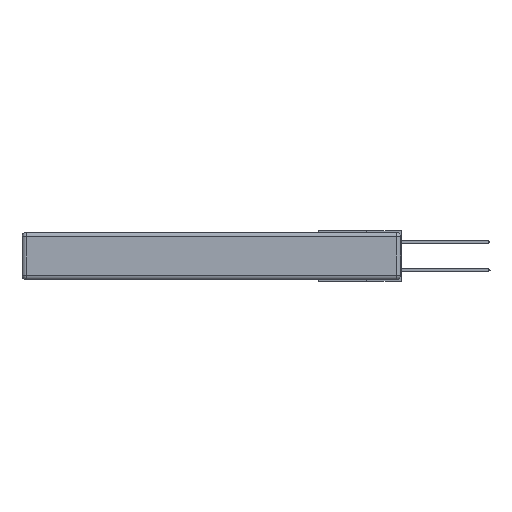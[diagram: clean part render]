
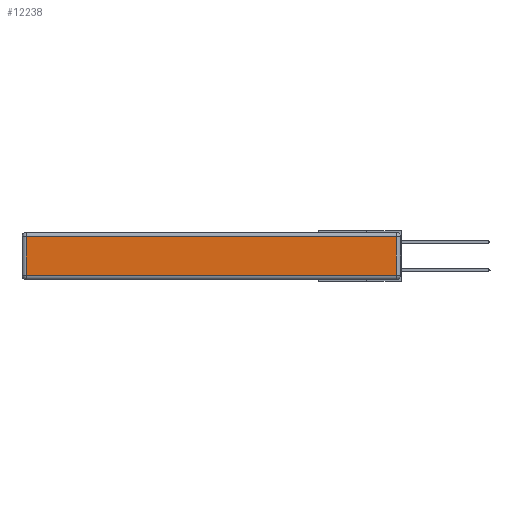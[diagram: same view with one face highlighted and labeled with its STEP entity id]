
A CAD part, left-side view. The second image highlights one B-rep face of the part: STEP entity #12238.
In plain terms, the highlighted planar face has unit normal (-1, 0, 0).
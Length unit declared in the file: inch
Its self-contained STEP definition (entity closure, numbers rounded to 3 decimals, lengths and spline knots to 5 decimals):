
#239 = DIRECTION ( 'NONE',  ( 0., 0., -1. ) ) ;
#331 = CARTESIAN_POINT ( 'NONE',  ( 0., 2.72, -0.313 ) ) ;
#1276 = VERTEX_POINT ( 'NONE', #11759 ) ;
#1335 = VECTOR ( 'NONE', #9742, 39.37008 ) ;
#1397 = CARTESIAN_POINT ( 'NONE',  ( 0., 0.03, -0.313 ) ) ;
#1874 = EDGE_CURVE ( 'NONE', #13864, #2983, #6659, .T. ) ;
#2343 = EDGE_LOOP ( 'NONE', ( #12414, #11600, #11601, #2745 ) ) ;
#2355 = AXIS2_PLACEMENT_3D ( 'NONE', #10193, #3668, #5344 ) ;
#2745 = ORIENTED_EDGE ( 'NONE', *, *, #7077, .T. ) ;
#2762 = VECTOR ( 'NONE', #4399, 39.37008 ) ;
#2983 = VERTEX_POINT ( 'NONE', #5739 ) ;
#3059 = CARTESIAN_POINT ( 'NONE',  ( 0., 0.03, -0.343 ) ) ;
#3190 = CARTESIAN_POINT ( 'NONE',  ( 0., 2.75, -0.03 ) ) ;
#3668 = DIRECTION ( 'NONE',  ( -1., 0., 0. ) ) ;
#4399 = DIRECTION ( 'NONE',  ( 0., -1., 0. ) ) ;
#5332 = FACE_OUTER_BOUND ( 'NONE', #2343, .T. ) ;
#5344 = DIRECTION ( 'NONE',  ( 0., 0., 1. ) ) ;
#5739 = CARTESIAN_POINT ( 'NONE',  ( 0., 0.03, -0.03 ) ) ;
#5845 = LINE ( 'NONE', #7852, #2762 ) ;
#6228 = VECTOR ( 'NONE', #9683, 39.37008 ) ;
#6659 = LINE ( 'NONE', #3059, #1335 ) ;
#7077 = EDGE_CURVE ( 'NONE', #1276, #11121, #7881, .T. ) ;
#7852 = CARTESIAN_POINT ( 'NONE',  ( 0., 0., -0.313 ) ) ;
#7881 = LINE ( 'NONE', #13876, #11560 ) ;
#8069 = PLANE ( 'NONE',  #2355 ) ;
#8637 = LINE ( 'NONE', #3190, #6228 ) ;
#9365 = EDGE_CURVE ( 'NONE', #2983, #1276, #8637, .T. ) ;
#9683 = DIRECTION ( 'NONE',  ( 0., 1., 0. ) ) ;
#9742 = DIRECTION ( 'NONE',  ( 0., 0., 1. ) ) ;
#10193 = CARTESIAN_POINT ( 'NONE',  ( 0., 0., -0.343 ) ) ;
#11121 = VERTEX_POINT ( 'NONE', #331 ) ;
#11560 = VECTOR ( 'NONE', #239, 39.37008 ) ;
#11600 = ORIENTED_EDGE ( 'NONE', *, *, #1874, .T. ) ;
#11601 = ORIENTED_EDGE ( 'NONE', *, *, #9365, .T. ) ;
#11759 = CARTESIAN_POINT ( 'NONE',  ( 0., 2.72, -0.03 ) ) ;
#12238 = ADVANCED_FACE ( 'NONE', ( #5332 ), #8069, .T. ) ;
#12297 = EDGE_CURVE ( 'NONE', #11121, #13864, #5845, .T. ) ;
#12414 = ORIENTED_EDGE ( 'NONE', *, *, #12297, .T. ) ;
#13864 = VERTEX_POINT ( 'NONE', #1397 ) ;
#13876 = CARTESIAN_POINT ( 'NONE',  ( 0., 2.72, -0.343 ) ) ;
